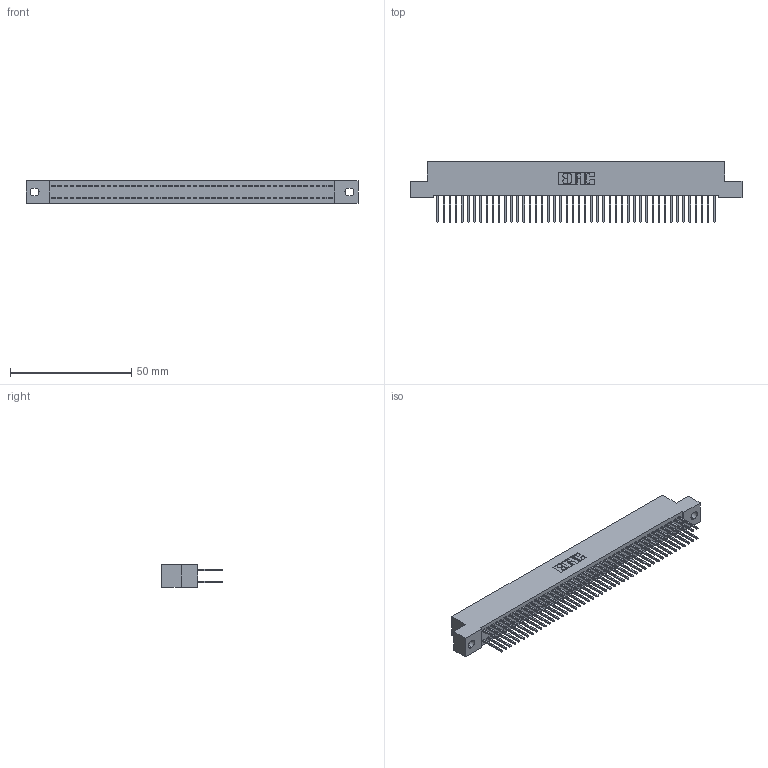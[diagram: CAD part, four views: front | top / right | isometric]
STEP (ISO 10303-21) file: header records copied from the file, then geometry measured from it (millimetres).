
FILE_DESCRIPTION (( 'STEP AP203' ), '1' );
FILE_NAME ('392-092-523-202.STEP', '2018-08-18T07:45:10', ( '' ), ( '' ), 'SwSTEP 2.0', 'SolidWorks 2016', '' );
FILE_SCHEMA (( 'CONFIG_CONTROL_DESIGN' ));
Length unit declared in the file: inch
Products named in the file (3): 342 Part_.128 Slot; 345-292-001_345-293-123; 392-092-523-202
Assembly tree (93 placements, depth 2):
  392-092-523-202
    342 Part_.128 Slot
    345-292-001_345-293-123  x92
Bounding box: 137.16 x 25.15 x 9.4 mm (x, y, z)
Volume: 12479.2 mm3; surface area: 20973.2 mm2
Topology: 93 solids, 93 shells, 4898 faces, 14571 edges, 9590 vertices
Faces by surface type: plane 3382, cylinder 1516
Entity records: 29097 total; most frequent: CARTESIAN_POINT 4818, ORIENTED_EDGE 4754, DIRECTION 4109, EDGE_CURVE 2377, VECTOR 2249, LINE 2249, VERTEX_POINT 1582, AXIS2_PLACEMENT_3D 930
